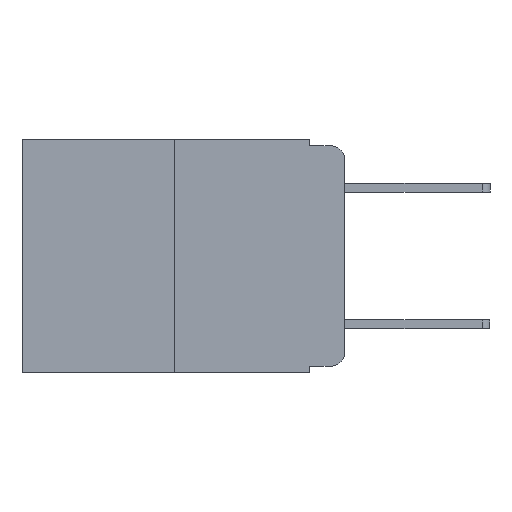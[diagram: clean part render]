
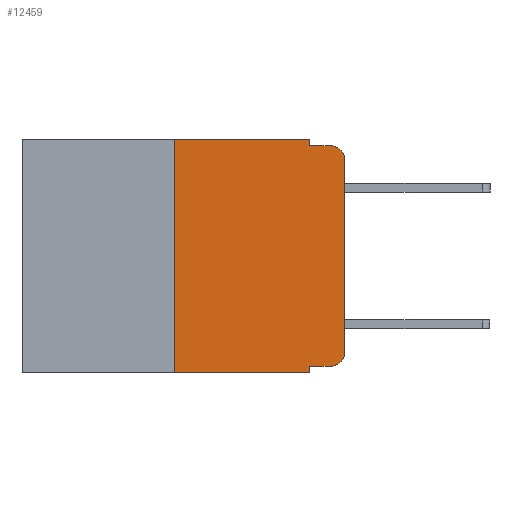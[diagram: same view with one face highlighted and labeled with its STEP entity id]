
A CAD part, left-side view. The second image highlights one B-rep face of the part: STEP entity #12459.
In plain terms, the highlighted planar face has unit normal (-1, 0, 0).
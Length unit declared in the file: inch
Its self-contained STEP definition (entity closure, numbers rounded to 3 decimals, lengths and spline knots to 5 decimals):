
#900 = VECTOR ( 'NONE', #8837, 39.37008 ) ;
#914 = DIRECTION ( 'NONE',  ( 0., -1., 0. ) ) ;
#1662 = ORIENTED_EDGE ( 'NONE', *, *, #2553, .F. ) ;
#1727 = VERTEX_POINT ( 'NONE', #5240 ) ;
#2553 = EDGE_CURVE ( 'NONE', #16458, #5760, #17986, .T. ) ;
#2608 = VERTEX_POINT ( 'NONE', #7293 ) ;
#2876 = CIRCLE ( 'NONE', #17015, 0.02 ) ;
#2970 = CARTESIAN_POINT ( 'NONE',  ( 0., 0.473, -0.343 ) ) ;
#3065 = AXIS2_PLACEMENT_3D ( 'NONE', #3518, #14814, #5257 ) ;
#3270 = ORIENTED_EDGE ( 'NONE', *, *, #19233, .F. ) ;
#3319 = CARTESIAN_POINT ( 'NONE',  ( 0., 0.051, -0.343 ) ) ;
#3518 = CARTESIAN_POINT ( 'NONE',  ( 0., 0.02, -0.03 ) ) ;
#4244 = DIRECTION ( 'NONE',  ( -1., 0., 0. ) ) ;
#4587 = CARTESIAN_POINT ( 'NONE',  ( 0., 0.473, 0. ) ) ;
#5240 = CARTESIAN_POINT ( 'NONE',  ( 0., 0.02, -0.01 ) ) ;
#5257 = DIRECTION ( 'NONE',  ( 0., 0., -1. ) ) ;
#5358 = VECTOR ( 'NONE', #914, 39.37008 ) ;
#5760 = VERTEX_POINT ( 'NONE', #15304 ) ;
#6187 = EDGE_LOOP ( 'NONE', ( #8563, #16855, #14161, #18280, #1662, #18752, #6763, #3270, #7754, #8304 ) ) ;
#6676 = EDGE_CURVE ( 'NONE', #10181, #15100, #2876, .T. ) ;
#6763 = ORIENTED_EDGE ( 'NONE', *, *, #13248, .T. ) ;
#7161 = CARTESIAN_POINT ( 'NONE',  ( 0., 0., 0. ) ) ;
#7293 = CARTESIAN_POINT ( 'NONE',  ( 0., 0.051, -0.333 ) ) ;
#7737 = EDGE_CURVE ( 'NONE', #2608, #10181, #20652, .T. ) ;
#7754 = ORIENTED_EDGE ( 'NONE', *, *, #7737, .T. ) ;
#7764 = VECTOR ( 'NONE', #17036, 39.37008 ) ;
#7941 = CARTESIAN_POINT ( 'NONE',  ( 0., 0.051, -0.01 ) ) ;
#8202 = DIRECTION ( 'NONE',  ( 0., 0., -1. ) ) ;
#8304 = ORIENTED_EDGE ( 'NONE', *, *, #6676, .T. ) ;
#8469 = AXIS2_PLACEMENT_3D ( 'NONE', #4587, #18870, #9640 ) ;
#8563 = ORIENTED_EDGE ( 'NONE', *, *, #15061, .T. ) ;
#8783 = CARTESIAN_POINT ( 'NONE',  ( 0., 0.25, 0. ) ) ;
#8837 = DIRECTION ( 'NONE',  ( 0., 0., 1. ) ) ;
#9261 = CARTESIAN_POINT ( 'NONE',  ( 0., 0.02, -0.333 ) ) ;
#9272 = LINE ( 'NONE', #17566, #13334 ) ;
#9276 = VECTOR ( 'NONE', #14402, 39.37008 ) ;
#9571 = PLANE ( 'NONE',  #8469 ) ;
#9640 = DIRECTION ( 'NONE',  ( 0., 0., -1. ) ) ;
#10093 = VERTEX_POINT ( 'NONE', #13621 ) ;
#10181 = VERTEX_POINT ( 'NONE', #9261 ) ;
#10235 = EDGE_CURVE ( 'NONE', #20265, #16458, #20130, .T. ) ;
#10425 = CARTESIAN_POINT ( 'NONE',  ( 0., 0., -0.313 ) ) ;
#10466 = CARTESIAN_POINT ( 'NONE',  ( 0., 0.473, 0. ) ) ;
#10701 = LINE ( 'NONE', #13326, #18421 ) ;
#10729 = FACE_OUTER_BOUND ( 'NONE', #6187, .T. ) ;
#10734 = LINE ( 'NONE', #7941, #14835 ) ;
#11815 = DIRECTION ( 'NONE',  ( 0., 0., -1. ) ) ;
#12459 = ADVANCED_FACE ( 'NONE', ( #10729 ), #9571, .F. ) ;
#12529 = EDGE_CURVE ( 'NONE', #5760, #10093, #9272, .T. ) ;
#12617 = VERTEX_POINT ( 'NONE', #3319 ) ;
#13164 = EDGE_CURVE ( 'NONE', #10093, #1727, #10734, .T. ) ;
#13248 = EDGE_CURVE ( 'NONE', #20265, #12617, #13338, .T. ) ;
#13326 = CARTESIAN_POINT ( 'NONE',  ( 0., 0.051, 0. ) ) ;
#13334 = VECTOR ( 'NONE', #8202, 39.37008 ) ;
#13338 = LINE ( 'NONE', #2970, #9276 ) ;
#13440 = EDGE_CURVE ( 'NONE', #15551, #1727, #14582, .T. ) ;
#13621 = CARTESIAN_POINT ( 'NONE',  ( 0., 0.051, -0.01 ) ) ;
#13886 = CARTESIAN_POINT ( 'NONE',  ( 0., 0.02, -0.313 ) ) ;
#14161 = ORIENTED_EDGE ( 'NONE', *, *, #13164, .F. ) ;
#14188 = DIRECTION ( 'NONE',  ( 0., -1., 0. ) ) ;
#14402 = DIRECTION ( 'NONE',  ( 0., -1., 0. ) ) ;
#14503 = CARTESIAN_POINT ( 'NONE',  ( 0., 0., -0.03 ) ) ;
#14582 = CIRCLE ( 'NONE', #3065, 0.02 ) ;
#14814 = DIRECTION ( 'NONE',  ( -1., 0., 0. ) ) ;
#14835 = VECTOR ( 'NONE', #18848, 39.37008 ) ;
#15061 = EDGE_CURVE ( 'NONE', #15100, #15551, #18151, .T. ) ;
#15100 = VERTEX_POINT ( 'NONE', #10425 ) ;
#15304 = CARTESIAN_POINT ( 'NONE',  ( 0., 0.051, 0. ) ) ;
#15488 = DIRECTION ( 'NONE',  ( 0., 0., -1. ) ) ;
#15551 = VERTEX_POINT ( 'NONE', #14503 ) ;
#15766 = CARTESIAN_POINT ( 'NONE',  ( 0., 0.051, -0.333 ) ) ;
#16227 = VECTOR ( 'NONE', #14188, 39.37008 ) ;
#16458 = VERTEX_POINT ( 'NONE', #8783 ) ;
#16855 = ORIENTED_EDGE ( 'NONE', *, *, #13440, .T. ) ;
#17015 = AXIS2_PLACEMENT_3D ( 'NONE', #13886, #4244, #15488 ) ;
#17036 = DIRECTION ( 'NONE',  ( 0., 0., 1. ) ) ;
#17548 = CARTESIAN_POINT ( 'NONE',  ( 0., 0.25, -0.343 ) ) ;
#17566 = CARTESIAN_POINT ( 'NONE',  ( 0., 0.051, 0. ) ) ;
#17986 = LINE ( 'NONE', #10466, #5358 ) ;
#18151 = LINE ( 'NONE', #7161, #900 ) ;
#18280 = ORIENTED_EDGE ( 'NONE', *, *, #12529, .F. ) ;
#18421 = VECTOR ( 'NONE', #11815, 39.37008 ) ;
#18562 = CARTESIAN_POINT ( 'NONE',  ( 0., 0.25, 0. ) ) ;
#18752 = ORIENTED_EDGE ( 'NONE', *, *, #10235, .F. ) ;
#18848 = DIRECTION ( 'NONE',  ( 0., -1., 0. ) ) ;
#18870 = DIRECTION ( 'NONE',  ( 1., 0., 0. ) ) ;
#19233 = EDGE_CURVE ( 'NONE', #2608, #12617, #10701, .T. ) ;
#20130 = LINE ( 'NONE', #18562, #7764 ) ;
#20265 = VERTEX_POINT ( 'NONE', #17548 ) ;
#20652 = LINE ( 'NONE', #15766, #16227 ) ;
